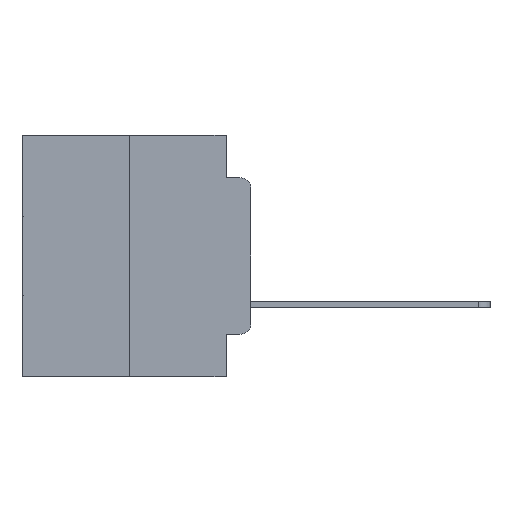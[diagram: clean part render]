
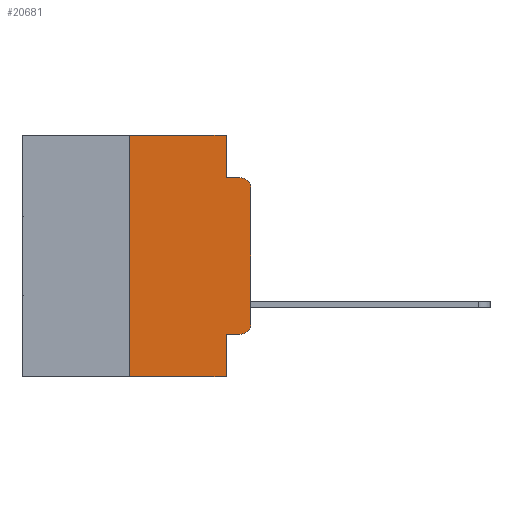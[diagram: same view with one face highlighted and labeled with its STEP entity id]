
A CAD part, left-side view. The second image highlights one B-rep face of the part: STEP entity #20681.
In plain terms, the highlighted planar face has unit normal (-1, 0, 0).
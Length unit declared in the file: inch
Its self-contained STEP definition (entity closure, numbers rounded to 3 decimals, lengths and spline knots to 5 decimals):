
#67 = LINE ( 'NONE', #7279, #18182 ) ;
#413 = LINE ( 'NONE', #6112, #12446 ) ;
#1171 = ORIENTED_EDGE ( 'NONE', *, *, #5113, .T. ) ;
#1192 = LINE ( 'NONE', #25499, #6883 ) ;
#1364 = ORIENTED_EDGE ( 'NONE', *, *, #29606, .T. ) ;
#1419 = PLANE ( 'NONE',  #5043 ) ;
#1555 = ORIENTED_EDGE ( 'NONE', *, *, #10277, .T. ) ;
#1669 = VECTOR ( 'NONE', #7716, 39.37008 ) ;
#2318 = CARTESIAN_POINT ( 'NONE',  ( 0., 0.473, -0.5 ) ) ;
#2997 = EDGE_CURVE ( 'NONE', #21085, #24156, #413, .T. ) ;
#3879 = DIRECTION ( 'NONE',  ( 0., 0., -1. ) ) ;
#4405 = CIRCLE ( 'NONE', #28572, 0.02 ) ;
#4720 = ORIENTED_EDGE ( 'NONE', *, *, #10325, .F. ) ;
#4788 = AXIS2_PLACEMENT_3D ( 'NONE', #27404, #14193, #29544 ) ;
#4877 = DIRECTION ( 'NONE',  ( 0., -1., 0. ) ) ;
#5043 = AXIS2_PLACEMENT_3D ( 'NONE', #8619, #17898, #3879 ) ;
#5092 = CARTESIAN_POINT ( 'NONE',  ( 0., 0., -0.1085 ) ) ;
#5113 = EDGE_CURVE ( 'NONE', #21938, #12944, #6275, .T. ) ;
#5546 = VECTOR ( 'NONE', #23033, 39.37008 ) ;
#6112 = CARTESIAN_POINT ( 'NONE',  ( 0., 0.051, 0. ) ) ;
#6275 = LINE ( 'NONE', #2318, #5546 ) ;
#6436 = VERTEX_POINT ( 'NONE', #20312 ) ;
#6691 = VERTEX_POINT ( 'NONE', #16803 ) ;
#6883 = VECTOR ( 'NONE', #27678, 39.37008 ) ;
#7006 = ORIENTED_EDGE ( 'NONE', *, *, #18651, .F. ) ;
#7279 = CARTESIAN_POINT ( 'NONE',  ( 0., 0.473, 0. ) ) ;
#7369 = ORIENTED_EDGE ( 'NONE', *, *, #21987, .T. ) ;
#7716 = DIRECTION ( 'NONE',  ( 0., -1., 0. ) ) ;
#8124 = ORIENTED_EDGE ( 'NONE', *, *, #9845, .T. ) ;
#8538 = DIRECTION ( 'NONE',  ( 0., 0., -1. ) ) ;
#8619 = CARTESIAN_POINT ( 'NONE',  ( 0., 0.473, 0. ) ) ;
#8647 = FACE_OUTER_BOUND ( 'NONE', #15584, .T. ) ;
#8799 = ORIENTED_EDGE ( 'NONE', *, *, #21070, .F. ) ;
#9545 = CARTESIAN_POINT ( 'NONE',  ( 0., 0.051, -0.0885 ) ) ;
#9845 = EDGE_CURVE ( 'NONE', #11720, #18979, #14339, .T. ) ;
#10125 = VECTOR ( 'NONE', #23658, 39.37008 ) ;
#10277 = EDGE_CURVE ( 'NONE', #27373, #6691, #20271, .T. ) ;
#10289 = DIRECTION ( 'NONE',  ( -1., 0., 0. ) ) ;
#10325 = EDGE_CURVE ( 'NONE', #14447, #21085, #67, .T. ) ;
#11720 = VERTEX_POINT ( 'NONE', #22618 ) ;
#11914 = CARTESIAN_POINT ( 'NONE',  ( 0., 0.051, -0.0885 ) ) ;
#12229 = CARTESIAN_POINT ( 'NONE',  ( 0., 0.25, -0.5 ) ) ;
#12446 = VECTOR ( 'NONE', #8538, 39.37008 ) ;
#12944 = VERTEX_POINT ( 'NONE', #20435 ) ;
#14193 = DIRECTION ( 'NONE',  ( -1., 0., 0. ) ) ;
#14339 = LINE ( 'NONE', #23638, #1669 ) ;
#14447 = VERTEX_POINT ( 'NONE', #16538 ) ;
#14728 = CARTESIAN_POINT ( 'NONE',  ( 0., 0.051, 0. ) ) ;
#15059 = LINE ( 'NONE', #27066, #26110 ) ;
#15584 = EDGE_LOOP ( 'NONE', ( #1364, #1555, #20318, #19960, #4720, #7006, #1171, #8799, #8124, #7369 ) ) ;
#16538 = CARTESIAN_POINT ( 'NONE',  ( 0., 0.25, 0. ) ) ;
#16803 = CARTESIAN_POINT ( 'NONE',  ( 0., 0.02, -0.0885 ) ) ;
#17898 = DIRECTION ( 'NONE',  ( 1., 0., 0. ) ) ;
#18182 = VECTOR ( 'NONE', #4877, 39.37008 ) ;
#18383 = LINE ( 'NONE', #9545, #29277 ) ;
#18646 = DIRECTION ( 'NONE',  ( 0., -1., 0. ) ) ;
#18651 = EDGE_CURVE ( 'NONE', #21938, #14447, #1192, .T. ) ;
#18979 = VERTEX_POINT ( 'NONE', #29254 ) ;
#19960 = ORIENTED_EDGE ( 'NONE', *, *, #2997, .F. ) ;
#20271 = CIRCLE ( 'NONE', #4788, 0.02 ) ;
#20312 = CARTESIAN_POINT ( 'NONE',  ( 0., 0., -0.3915 ) ) ;
#20318 = ORIENTED_EDGE ( 'NONE', *, *, #26516, .F. ) ;
#20435 = CARTESIAN_POINT ( 'NONE',  ( 0., 0.051, -0.5 ) ) ;
#20681 = ADVANCED_FACE ( 'NONE', ( #8647 ), #1419, .F. ) ;
#21070 = EDGE_CURVE ( 'NONE', #11720, #12944, #27905, .T. ) ;
#21085 = VERTEX_POINT ( 'NONE', #14728 ) ;
#21466 = CARTESIAN_POINT ( 'NONE',  ( 0., 0.051, 0. ) ) ;
#21938 = VERTEX_POINT ( 'NONE', #12229 ) ;
#21987 = EDGE_CURVE ( 'NONE', #18979, #6436, #4405, .T. ) ;
#22618 = CARTESIAN_POINT ( 'NONE',  ( 0., 0.051, -0.4115 ) ) ;
#23033 = DIRECTION ( 'NONE',  ( 0., -1., 0. ) ) ;
#23638 = CARTESIAN_POINT ( 'NONE',  ( 0., 0.051, -0.4115 ) ) ;
#23658 = DIRECTION ( 'NONE',  ( 0., 0., -1. ) ) ;
#23755 = CARTESIAN_POINT ( 'NONE',  ( 0., 0.02, -0.3915 ) ) ;
#24156 = VERTEX_POINT ( 'NONE', #11914 ) ;
#25499 = CARTESIAN_POINT ( 'NONE',  ( 0., 0.25, 0. ) ) ;
#25923 = DIRECTION ( 'NONE',  ( 0., 0., -1. ) ) ;
#26110 = VECTOR ( 'NONE', #29211, 39.37008 ) ;
#26516 = EDGE_CURVE ( 'NONE', #24156, #6691, #18383, .T. ) ;
#27066 = CARTESIAN_POINT ( 'NONE',  ( 0., 0., 0. ) ) ;
#27373 = VERTEX_POINT ( 'NONE', #5092 ) ;
#27404 = CARTESIAN_POINT ( 'NONE',  ( 0., 0.02, -0.1085 ) ) ;
#27678 = DIRECTION ( 'NONE',  ( 0., 0., 1. ) ) ;
#27905 = LINE ( 'NONE', #21466, #10125 ) ;
#28572 = AXIS2_PLACEMENT_3D ( 'NONE', #23755, #10289, #25923 ) ;
#29211 = DIRECTION ( 'NONE',  ( 0., 0., 1. ) ) ;
#29254 = CARTESIAN_POINT ( 'NONE',  ( 0., 0.02, -0.4115 ) ) ;
#29277 = VECTOR ( 'NONE', #18646, 39.37008 ) ;
#29544 = DIRECTION ( 'NONE',  ( 0., 0., -1. ) ) ;
#29606 = EDGE_CURVE ( 'NONE', #6436, #27373, #15059, .T. ) ;
